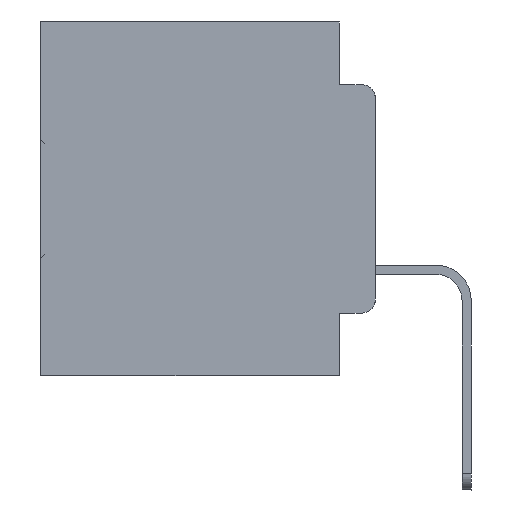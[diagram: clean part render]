
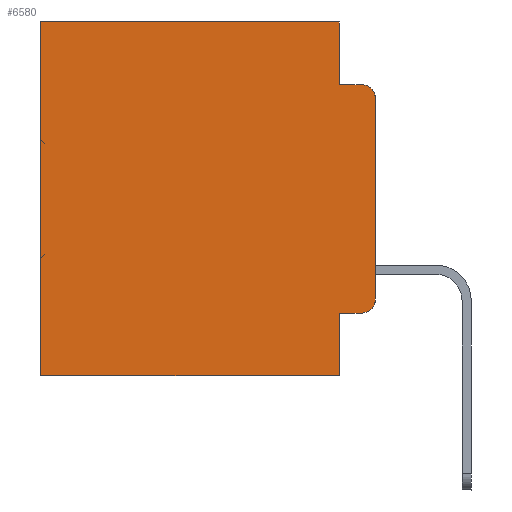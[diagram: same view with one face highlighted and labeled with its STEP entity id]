
A CAD part, left-side view. The second image highlights one B-rep face of the part: STEP entity #6580.
In plain terms, the highlighted planar face has unit normal (-1, 0, 0).
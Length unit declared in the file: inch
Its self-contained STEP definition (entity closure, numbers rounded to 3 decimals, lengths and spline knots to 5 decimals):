
#122 = EDGE_CURVE ( 'NONE', #13442, #22665, #20519, .T. ) ;
#322 = DIRECTION ( 'NONE',  ( 0., 0., -1. ) ) ;
#945 = CARTESIAN_POINT ( 'NONE',  ( 0.298, 0.051, -0.4115 ) ) ;
#1183 = DIRECTION ( 'NONE',  ( 0., 1., 0. ) ) ;
#1305 = EDGE_CURVE ( 'NONE', #13271, #20031, #11471, .T. ) ;
#1447 = LINE ( 'NONE', #21668, #7799 ) ;
#1814 = CARTESIAN_POINT ( 'NONE',  ( 0.298, 0.051, -0.5 ) ) ;
#3909 = DIRECTION ( 'NONE',  ( 0., -1., 0. ) ) ;
#4459 = VERTEX_POINT ( 'NONE', #6302 ) ;
#5269 = ORIENTED_EDGE ( 'NONE', *, *, #20593, .T. ) ;
#5370 = ORIENTED_EDGE ( 'NONE', *, *, #15255, .F. ) ;
#5669 = ORIENTED_EDGE ( 'NONE', *, *, #23711, .T. ) ;
#6040 = DIRECTION ( 'NONE',  ( 0., 0., -1. ) ) ;
#6254 = VERTEX_POINT ( 'NONE', #15908 ) ;
#6302 = CARTESIAN_POINT ( 'NONE',  ( 0.298, 0.051, -0.0885 ) ) ;
#6580 = ADVANCED_FACE ( 'NONE', ( #14891 ), #16929, .F. ) ;
#7614 = LINE ( 'NONE', #8007, #34294 ) ;
#7678 = DIRECTION ( 'NONE',  ( 0., 1., 0. ) ) ;
#7799 = VECTOR ( 'NONE', #6040, 39.37008 ) ;
#8007 = CARTESIAN_POINT ( 'NONE',  ( 0.298, 0., -0.5 ) ) ;
#8828 = CARTESIAN_POINT ( 'NONE',  ( 0.298, 0., -0.1085 ) ) ;
#9088 = LINE ( 'NONE', #34082, #20513 ) ;
#9354 = CARTESIAN_POINT ( 'NONE',  ( 0.298, 0.051, -0.4115 ) ) ;
#10001 = VECTOR ( 'NONE', #31286, 39.37008 ) ;
#11471 = LINE ( 'NONE', #33623, #21583 ) ;
#12362 = CARTESIAN_POINT ( 'NONE',  ( 0.298, 0.473, -0.5 ) ) ;
#12841 = EDGE_CURVE ( 'NONE', #14532, #6254, #23168, .T. ) ;
#13271 = VERTEX_POINT ( 'NONE', #29788 ) ;
#13442 = VERTEX_POINT ( 'NONE', #8828 ) ;
#13770 = ORIENTED_EDGE ( 'NONE', *, *, #19605, .F. ) ;
#14532 = VERTEX_POINT ( 'NONE', #945 ) ;
#14822 = DIRECTION ( 'NONE',  ( 0., 0., -1. ) ) ;
#14891 = FACE_OUTER_BOUND ( 'NONE', #33719, .T. ) ;
#15255 = EDGE_CURVE ( 'NONE', #14532, #18333, #20336, .T. ) ;
#15366 = CARTESIAN_POINT ( 'NONE',  ( 0.298, 0.051, 0. ) ) ;
#15908 = CARTESIAN_POINT ( 'NONE',  ( 0.298, 0.02, -0.4115 ) ) ;
#16864 = ORIENTED_EDGE ( 'NONE', *, *, #31433, .F. ) ;
#16881 = ORIENTED_EDGE ( 'NONE', *, *, #28746, .F. ) ;
#16929 = PLANE ( 'NONE',  #29856 ) ;
#17912 = DIRECTION ( 'NONE',  ( 0., 0., -1. ) ) ;
#18333 = VERTEX_POINT ( 'NONE', #1814 ) ;
#18631 = CARTESIAN_POINT ( 'NONE',  ( 0.298, 0.02, -0.1085 ) ) ;
#18827 = LINE ( 'NONE', #30479, #33670 ) ;
#19274 = CARTESIAN_POINT ( 'NONE',  ( 0.298, 0.02, -0.3915 ) ) ;
#19511 = DIRECTION ( 'NONE',  ( -1., 0., 0. ) ) ;
#19605 = EDGE_CURVE ( 'NONE', #4459, #22665, #18827, .T. ) ;
#19651 = ORIENTED_EDGE ( 'NONE', *, *, #12841, .T. ) ;
#19726 = DIRECTION ( 'NONE',  ( 0., -1., 0. ) ) ;
#20031 = VERTEX_POINT ( 'NONE', #21114 ) ;
#20336 = LINE ( 'NONE', #33925, #29198 ) ;
#20513 = VECTOR ( 'NONE', #17912, 39.37008 ) ;
#20519 = CIRCLE ( 'NONE', #22218, 0.02 ) ;
#20593 = EDGE_CURVE ( 'NONE', #20031, #25337, #9088, .T. ) ;
#21114 = CARTESIAN_POINT ( 'NONE',  ( 0.298, 0.473, 0. ) ) ;
#21583 = VECTOR ( 'NONE', #1183, 39.37008 ) ;
#21668 = CARTESIAN_POINT ( 'NONE',  ( 0.298, 0., 0. ) ) ;
#21688 = DIRECTION ( 'NONE',  ( -1., 0., 0. ) ) ;
#22218 = AXIS2_PLACEMENT_3D ( 'NONE', #18631, #21688, #27104 ) ;
#22665 = VERTEX_POINT ( 'NONE', #33282 ) ;
#23168 = LINE ( 'NONE', #9354, #28679 ) ;
#23711 = EDGE_CURVE ( 'NONE', #6254, #28451, #26987, .T. ) ;
#23921 = LINE ( 'NONE', #15366, #10001 ) ;
#25337 = VERTEX_POINT ( 'NONE', #12362 ) ;
#26987 = CIRCLE ( 'NONE', #31824, 0.02 ) ;
#27104 = DIRECTION ( 'NONE',  ( 0., 0., -1. ) ) ;
#27538 = CARTESIAN_POINT ( 'NONE',  ( 0.298, 0., 0. ) ) ;
#28451 = VERTEX_POINT ( 'NONE', #31283 ) ;
#28679 = VECTOR ( 'NONE', #3909, 39.37008 ) ;
#28746 = EDGE_CURVE ( 'NONE', #13442, #28451, #1447, .T. ) ;
#29019 = ORIENTED_EDGE ( 'NONE', *, *, #32381, .F. ) ;
#29198 = VECTOR ( 'NONE', #14822, 39.37008 ) ;
#29788 = CARTESIAN_POINT ( 'NONE',  ( 0.298, 0.051, 0. ) ) ;
#29856 = AXIS2_PLACEMENT_3D ( 'NONE', #27538, #33226, #322 ) ;
#30139 = DIRECTION ( 'NONE',  ( 0., 0., -1. ) ) ;
#30192 = ORIENTED_EDGE ( 'NONE', *, *, #122, .T. ) ;
#30479 = CARTESIAN_POINT ( 'NONE',  ( 0.298, 0.051, -0.0885 ) ) ;
#31283 = CARTESIAN_POINT ( 'NONE',  ( 0.298, 0., -0.3915 ) ) ;
#31286 = DIRECTION ( 'NONE',  ( 0., 0., -1. ) ) ;
#31433 = EDGE_CURVE ( 'NONE', #18333, #25337, #7614, .T. ) ;
#31824 = AXIS2_PLACEMENT_3D ( 'NONE', #19274, #19511, #30139 ) ;
#32364 = ORIENTED_EDGE ( 'NONE', *, *, #1305, .T. ) ;
#32381 = EDGE_CURVE ( 'NONE', #13271, #4459, #23921, .T. ) ;
#33226 = DIRECTION ( 'NONE',  ( 1., 0., 0. ) ) ;
#33282 = CARTESIAN_POINT ( 'NONE',  ( 0.298, 0.02, -0.0885 ) ) ;
#33623 = CARTESIAN_POINT ( 'NONE',  ( 0.298, 0., 0. ) ) ;
#33670 = VECTOR ( 'NONE', #19726, 39.37008 ) ;
#33719 = EDGE_LOOP ( 'NONE', ( #16881, #30192, #13770, #29019, #32364, #5269, #16864, #5370, #19651, #5669 ) ) ;
#33925 = CARTESIAN_POINT ( 'NONE',  ( 0.298, 0.051, 0. ) ) ;
#34082 = CARTESIAN_POINT ( 'NONE',  ( 0.298, 0.473, 0. ) ) ;
#34294 = VECTOR ( 'NONE', #7678, 39.37008 ) ;
